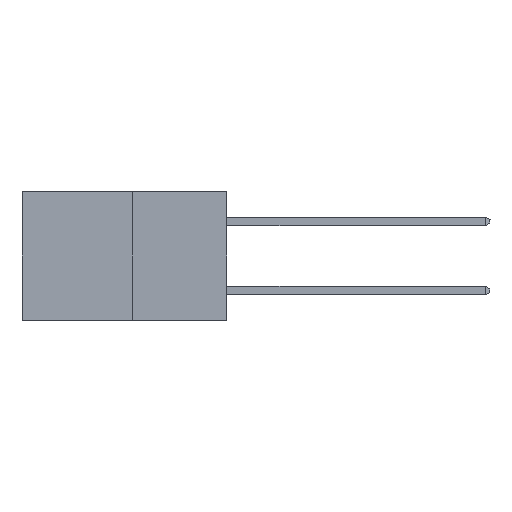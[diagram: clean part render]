
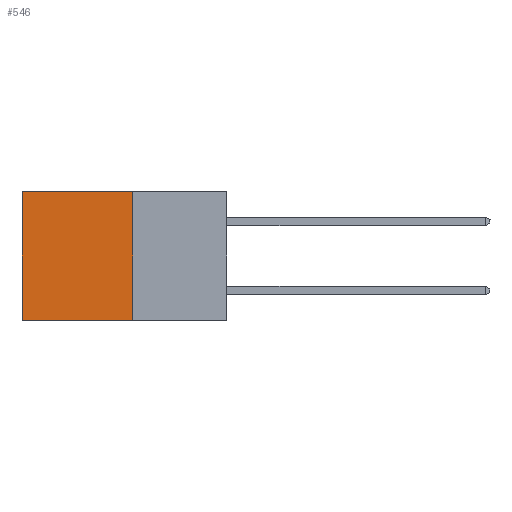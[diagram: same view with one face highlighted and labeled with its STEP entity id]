
A CAD part, left-side view. The second image highlights one B-rep face of the part: STEP entity #546.
In plain terms, the highlighted planar face has unit normal (-1, 0, 0).
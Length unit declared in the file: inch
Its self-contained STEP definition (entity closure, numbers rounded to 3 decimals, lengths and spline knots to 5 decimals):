
#534 = EDGE_CURVE ( 'NONE', #10943, #8469, #12074, .T. ) ;
#546 = ADVANCED_FACE ( 'NONE', ( #9540 ), #7699, .F. ) ;
#720 = CARTESIAN_POINT ( 'NONE',  ( 0.277, 0.27, 0. ) ) ;
#754 = VERTEX_POINT ( 'NONE', #9961 ) ;
#813 = VECTOR ( 'NONE', #2639, 39.37008 ) ;
#2099 = LINE ( 'NONE', #9083, #7211 ) ;
#2639 = DIRECTION ( 'NONE',  ( 0., 1., 0. ) ) ;
#3035 = CARTESIAN_POINT ( 'NONE',  ( 0.277, 0.27, -0.37 ) ) ;
#3845 = ORIENTED_EDGE ( 'NONE', *, *, #4345, .F. ) ;
#4345 = EDGE_CURVE ( 'NONE', #8469, #12583, #7050, .T. ) ;
#5141 = CARTESIAN_POINT ( 'NONE',  ( 0.277, 0.27, -0.37 ) ) ;
#5590 = CARTESIAN_POINT ( 'NONE',  ( 0.277, 0.27, -0.37 ) ) ;
#5886 = EDGE_LOOP ( 'NONE', ( #7724, #3845, #10646, #9109 ) ) ;
#6000 = DIRECTION ( 'NONE',  ( 0., 0., -1. ) ) ;
#6366 = LINE ( 'NONE', #720, #813 ) ;
#6752 = VECTOR ( 'NONE', #8427, 39.37008 ) ;
#7050 = LINE ( 'NONE', #7321, #6752 ) ;
#7211 = VECTOR ( 'NONE', #8132, 39.37008 ) ;
#7321 = CARTESIAN_POINT ( 'NONE',  ( 0.277, 0.27, -0.37 ) ) ;
#7699 = PLANE ( 'NONE',  #8693 ) ;
#7724 = ORIENTED_EDGE ( 'NONE', *, *, #11551, .T. ) ;
#8056 = EDGE_CURVE ( 'NONE', #10943, #754, #6366, .T. ) ;
#8132 = DIRECTION ( 'NONE',  ( 0., 0., -1. ) ) ;
#8427 = DIRECTION ( 'NONE',  ( 0., 1., 0. ) ) ;
#8469 = VERTEX_POINT ( 'NONE', #5141 ) ;
#8693 = AXIS2_PLACEMENT_3D ( 'NONE', #3035, #12328, #9599 ) ;
#9083 = CARTESIAN_POINT ( 'NONE',  ( 0.277, 0.59, -0.37 ) ) ;
#9095 = CARTESIAN_POINT ( 'NONE',  ( 0.277, 0.59, -0.37 ) ) ;
#9109 = ORIENTED_EDGE ( 'NONE', *, *, #8056, .T. ) ;
#9182 = CARTESIAN_POINT ( 'NONE',  ( 0.277, 0.27, 0. ) ) ;
#9540 = FACE_OUTER_BOUND ( 'NONE', #5886, .T. ) ;
#9599 = DIRECTION ( 'NONE',  ( 0., 0., -1. ) ) ;
#9850 = VECTOR ( 'NONE', #6000, 39.37008 ) ;
#9961 = CARTESIAN_POINT ( 'NONE',  ( 0.277, 0.59, 0. ) ) ;
#10646 = ORIENTED_EDGE ( 'NONE', *, *, #534, .F. ) ;
#10943 = VERTEX_POINT ( 'NONE', #9182 ) ;
#11551 = EDGE_CURVE ( 'NONE', #754, #12583, #2099, .T. ) ;
#12074 = LINE ( 'NONE', #5590, #9850 ) ;
#12328 = DIRECTION ( 'NONE',  ( 1., 0., 0. ) ) ;
#12583 = VERTEX_POINT ( 'NONE', #9095 ) ;
